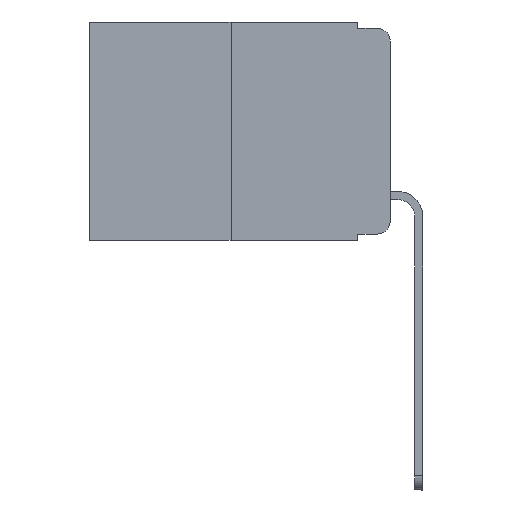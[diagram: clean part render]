
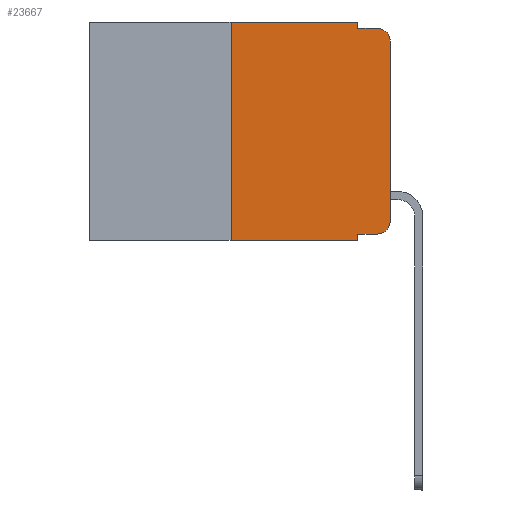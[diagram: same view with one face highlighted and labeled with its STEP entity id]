
A CAD part, left-side view. The second image highlights one B-rep face of the part: STEP entity #23667.
In plain terms, the highlighted planar face has unit normal (-1, 0, 0).
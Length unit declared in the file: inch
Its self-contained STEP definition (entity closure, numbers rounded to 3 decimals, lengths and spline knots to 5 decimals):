
#245 = ORIENTED_EDGE ( 'NONE', *, *, #19767, .T. ) ;
#310 = ORIENTED_EDGE ( 'NONE', *, *, #1130, .F. ) ;
#352 = PLANE ( 'NONE',  #12863 ) ;
#586 = DIRECTION ( 'NONE',  ( 0., 0., 1. ) ) ;
#966 = CARTESIAN_POINT ( 'NONE',  ( 0., 0.051, -0.333 ) ) ;
#1130 = EDGE_CURVE ( 'NONE', #3760, #1752, #3233, .T. ) ;
#1170 = DIRECTION ( 'NONE',  ( 0., 0., -1. ) ) ;
#1180 = EDGE_CURVE ( 'NONE', #19278, #1752, #13110, .T. ) ;
#1459 = LINE ( 'NONE', #17061, #13934 ) ;
#1579 = AXIS2_PLACEMENT_3D ( 'NONE', #9280, #23358, #1170 ) ;
#1650 = CARTESIAN_POINT ( 'NONE',  ( 0., 0., 0. ) ) ;
#1752 = VERTEX_POINT ( 'NONE', #15703 ) ;
#1800 = VECTOR ( 'NONE', #5891, 39.37008 ) ;
#1859 = CARTESIAN_POINT ( 'NONE',  ( 0., 0.25, -0.343 ) ) ;
#2559 = FACE_OUTER_BOUND ( 'NONE', #5958, .T. ) ;
#2903 = ORIENTED_EDGE ( 'NONE', *, *, #6884, .T. ) ;
#3169 = AXIS2_PLACEMENT_3D ( 'NONE', #7532, #5217, #11156 ) ;
#3206 = VERTEX_POINT ( 'NONE', #19119 ) ;
#3233 = LINE ( 'NONE', #11087, #4860 ) ;
#3582 = EDGE_CURVE ( 'NONE', #14602, #3206, #23220, .T. ) ;
#3760 = VERTEX_POINT ( 'NONE', #15720 ) ;
#4236 = EDGE_CURVE ( 'NONE', #14293, #14602, #22394, .T. ) ;
#4568 = ORIENTED_EDGE ( 'NONE', *, *, #3582, .F. ) ;
#4597 = ORIENTED_EDGE ( 'NONE', *, *, #4236, .F. ) ;
#4652 = LINE ( 'NONE', #1650, #8500 ) ;
#4860 = VECTOR ( 'NONE', #5529, 39.37008 ) ;
#5217 = DIRECTION ( 'NONE',  ( -1., 0., 0. ) ) ;
#5231 = CARTESIAN_POINT ( 'NONE',  ( 0., 0., -0.313 ) ) ;
#5394 = DIRECTION ( 'NONE',  ( 0., -1., 0. ) ) ;
#5529 = DIRECTION ( 'NONE',  ( 0., -1., 0. ) ) ;
#5737 = ORIENTED_EDGE ( 'NONE', *, *, #1180, .T. ) ;
#5891 = DIRECTION ( 'NONE',  ( 0., -1., 0. ) ) ;
#5958 = EDGE_LOOP ( 'NONE', ( #11343, #5737, #310, #10447, #4568, #4597, #12815, #8977, #245, #2903 ) ) ;
#6273 = CARTESIAN_POINT ( 'NONE',  ( 0., 0.473, 0. ) ) ;
#6838 = CARTESIAN_POINT ( 'NONE',  ( 0., 0.051, -0.343 ) ) ;
#6884 = EDGE_CURVE ( 'NONE', #7376, #15778, #23762, .T. ) ;
#6944 = CARTESIAN_POINT ( 'NONE',  ( 0., 0., -0.03 ) ) ;
#7376 = VERTEX_POINT ( 'NONE', #13050 ) ;
#7532 = CARTESIAN_POINT ( 'NONE',  ( 0., 0.02, -0.313 ) ) ;
#8310 = VERTEX_POINT ( 'NONE', #966 ) ;
#8500 = VECTOR ( 'NONE', #9639, 39.37008 ) ;
#8777 = VECTOR ( 'NONE', #19899, 39.37008 ) ;
#8977 = ORIENTED_EDGE ( 'NONE', *, *, #24245, .F. ) ;
#9280 = CARTESIAN_POINT ( 'NONE',  ( 0., 0.02, -0.03 ) ) ;
#9639 = DIRECTION ( 'NONE',  ( 0., 0., 1. ) ) ;
#10252 = CARTESIAN_POINT ( 'NONE',  ( 0., 0.051, -0.333 ) ) ;
#10447 = ORIENTED_EDGE ( 'NONE', *, *, #17945, .F. ) ;
#11074 = CARTESIAN_POINT ( 'NONE',  ( 0., 0.473, 0. ) ) ;
#11087 = CARTESIAN_POINT ( 'NONE',  ( 0., 0.051, -0.01 ) ) ;
#11156 = DIRECTION ( 'NONE',  ( 0., 0., -1. ) ) ;
#11343 = ORIENTED_EDGE ( 'NONE', *, *, #12086, .T. ) ;
#12086 = EDGE_CURVE ( 'NONE', #15778, #19278, #4652, .T. ) ;
#12101 = DIRECTION ( 'NONE',  ( 0., 0., -1. ) ) ;
#12299 = VECTOR ( 'NONE', #15921, 39.37008 ) ;
#12815 = ORIENTED_EDGE ( 'NONE', *, *, #13987, .T. ) ;
#12863 = AXIS2_PLACEMENT_3D ( 'NONE', #6273, #20839, #12101 ) ;
#13037 = CARTESIAN_POINT ( 'NONE',  ( 0., 0.25, 0. ) ) ;
#13050 = CARTESIAN_POINT ( 'NONE',  ( 0., 0.02, -0.333 ) ) ;
#13060 = DIRECTION ( 'NONE',  ( 0., 0., -1. ) ) ;
#13110 = CIRCLE ( 'NONE', #1579, 0.02 ) ;
#13934 = VECTOR ( 'NONE', #13060, 39.37008 ) ;
#13987 = EDGE_CURVE ( 'NONE', #14293, #21716, #25398, .T. ) ;
#14293 = VERTEX_POINT ( 'NONE', #1859 ) ;
#14389 = CARTESIAN_POINT ( 'NONE',  ( 0., 0.25, 0. ) ) ;
#14602 = VERTEX_POINT ( 'NONE', #13037 ) ;
#15703 = CARTESIAN_POINT ( 'NONE',  ( 0., 0.02, -0.01 ) ) ;
#15720 = CARTESIAN_POINT ( 'NONE',  ( 0., 0.051, -0.01 ) ) ;
#15748 = CARTESIAN_POINT ( 'NONE',  ( 0., 0.051, 0. ) ) ;
#15778 = VERTEX_POINT ( 'NONE', #5231 ) ;
#15921 = DIRECTION ( 'NONE',  ( 0., -1., 0. ) ) ;
#17061 = CARTESIAN_POINT ( 'NONE',  ( 0., 0.051, 0. ) ) ;
#17875 = LINE ( 'NONE', #10252, #12299 ) ;
#17945 = EDGE_CURVE ( 'NONE', #3206, #3760, #1459, .T. ) ;
#19119 = CARTESIAN_POINT ( 'NONE',  ( 0., 0.051, 0. ) ) ;
#19278 = VERTEX_POINT ( 'NONE', #6944 ) ;
#19767 = EDGE_CURVE ( 'NONE', #8310, #7376, #17875, .T. ) ;
#19854 = CARTESIAN_POINT ( 'NONE',  ( 0., 0.473, -0.343 ) ) ;
#19899 = DIRECTION ( 'NONE',  ( 0., 0., -1. ) ) ;
#20839 = DIRECTION ( 'NONE',  ( 1., 0., 0. ) ) ;
#21716 = VERTEX_POINT ( 'NONE', #6838 ) ;
#22394 = LINE ( 'NONE', #14389, #24029 ) ;
#23220 = LINE ( 'NONE', #11074, #24790 ) ;
#23358 = DIRECTION ( 'NONE',  ( -1., 0., 0. ) ) ;
#23667 = ADVANCED_FACE ( 'NONE', ( #2559 ), #352, .F. ) ;
#23762 = CIRCLE ( 'NONE', #3169, 0.02 ) ;
#24029 = VECTOR ( 'NONE', #586, 39.37008 ) ;
#24245 = EDGE_CURVE ( 'NONE', #8310, #21716, #25185, .T. ) ;
#24790 = VECTOR ( 'NONE', #5394, 39.37008 ) ;
#25185 = LINE ( 'NONE', #15748, #8777 ) ;
#25398 = LINE ( 'NONE', #19854, #1800 ) ;
